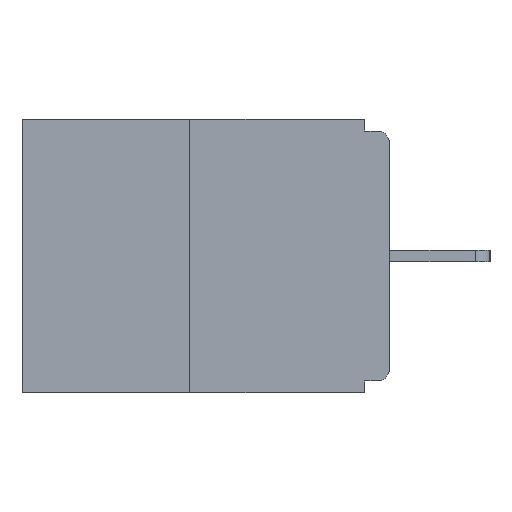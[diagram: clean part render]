
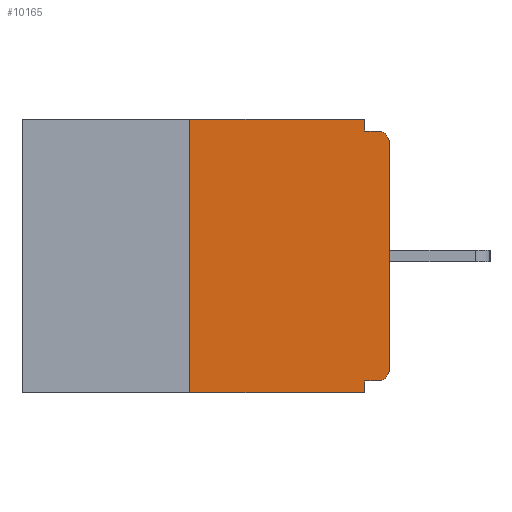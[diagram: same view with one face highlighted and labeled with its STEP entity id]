
A CAD part, left-side view. The second image highlights one B-rep face of the part: STEP entity #10165.
In plain terms, the highlighted planar face has unit normal (-1, 0, 0).
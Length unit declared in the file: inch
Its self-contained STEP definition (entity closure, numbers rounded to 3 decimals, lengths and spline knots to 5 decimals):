
#77 = CARTESIAN_POINT ( 'NONE',  ( 0., 0.031, -0.343 ) ) ;
#112 = LINE ( 'NONE', #6906, #4555 ) ;
#168 = CARTESIAN_POINT ( 'NONE',  ( 0., 0.015, -0.03 ) ) ;
#309 = EDGE_CURVE ( 'NONE', #3891, #2031, #1038, .T. ) ;
#332 = DIRECTION ( 'NONE',  ( 0., 0., -1. ) ) ;
#1038 = LINE ( 'NONE', #4502, #12500 ) ;
#1182 = DIRECTION ( 'NONE',  ( 0., 0., -1. ) ) ;
#1231 = LINE ( 'NONE', #9130, #6638 ) ;
#1246 = EDGE_CURVE ( 'NONE', #8167, #6120, #4757, .T. ) ;
#1409 = ORIENTED_EDGE ( 'NONE', *, *, #309, .F. ) ;
#1579 = CARTESIAN_POINT ( 'NONE',  ( 0., 0., -0.328 ) ) ;
#1646 = VECTOR ( 'NONE', #14149, 39.37008 ) ;
#2031 = VERTEX_POINT ( 'NONE', #12581 ) ;
#2086 = CARTESIAN_POINT ( 'NONE',  ( 0., 0., -0.015 ) ) ;
#2393 = CARTESIAN_POINT ( 'NONE',  ( 0., 0.25, 0. ) ) ;
#2435 = ORIENTED_EDGE ( 'NONE', *, *, #1246, .T. ) ;
#2538 = DIRECTION ( 'NONE',  ( 0., 0., -1. ) ) ;
#2892 = EDGE_CURVE ( 'NONE', #6120, #8867, #10414, .T. ) ;
#3106 = LINE ( 'NONE', #6288, #1646 ) ;
#3425 = CARTESIAN_POINT ( 'NONE',  ( 0., 0.015, -0.328 ) ) ;
#3812 = EDGE_CURVE ( 'NONE', #9944, #8167, #5420, .T. ) ;
#3814 = ORIENTED_EDGE ( 'NONE', *, *, #2892, .T. ) ;
#3891 = VERTEX_POINT ( 'NONE', #12996 ) ;
#4291 = CARTESIAN_POINT ( 'NONE',  ( 0., 0.25, -0.343 ) ) ;
#4444 = CARTESIAN_POINT ( 'NONE',  ( 0., 0.46, 0. ) ) ;
#4502 = CARTESIAN_POINT ( 'NONE',  ( 0., 0.031, 0. ) ) ;
#4518 = ORIENTED_EDGE ( 'NONE', *, *, #3812, .T. ) ;
#4555 = VECTOR ( 'NONE', #4827, 39.37008 ) ;
#4739 = AXIS2_PLACEMENT_3D ( 'NONE', #168, #8147, #2538 ) ;
#4757 = LINE ( 'NONE', #8087, #12994 ) ;
#4827 = DIRECTION ( 'NONE',  ( 0., -1., 0. ) ) ;
#4846 = CARTESIAN_POINT ( 'NONE',  ( 0., 0.031, -0.328 ) ) ;
#5420 = CIRCLE ( 'NONE', #14435, 0.015 ) ;
#5537 = EDGE_CURVE ( 'NONE', #14638, #13087, #3106, .T. ) ;
#6006 = VECTOR ( 'NONE', #13215, 39.37008 ) ;
#6070 = ORIENTED_EDGE ( 'NONE', *, *, #12764, .T. ) ;
#6120 = VERTEX_POINT ( 'NONE', #12477 ) ;
#6288 = CARTESIAN_POINT ( 'NONE',  ( 0., 0.25, 0. ) ) ;
#6302 = DIRECTION ( 'NONE',  ( -1., 0., 0. ) ) ;
#6491 = ORIENTED_EDGE ( 'NONE', *, *, #8341, .F. ) ;
#6595 = LINE ( 'NONE', #4444, #7169 ) ;
#6638 = VECTOR ( 'NONE', #332, 39.37008 ) ;
#6906 = CARTESIAN_POINT ( 'NONE',  ( 0., 0.46, -0.343 ) ) ;
#7099 = LINE ( 'NONE', #1579, #7656 ) ;
#7163 = EDGE_LOOP ( 'NONE', ( #13768, #14535, #6070, #6491, #8453, #4518, #2435, #3814, #11019, #1409 ) ) ;
#7169 = VECTOR ( 'NONE', #13229, 39.37008 ) ;
#7449 = VERTEX_POINT ( 'NONE', #77 ) ;
#7656 = VECTOR ( 'NONE', #13795, 39.37008 ) ;
#8087 = CARTESIAN_POINT ( 'NONE',  ( 0., 0., 0. ) ) ;
#8147 = DIRECTION ( 'NONE',  ( -1., 0., 0. ) ) ;
#8167 = VERTEX_POINT ( 'NONE', #11284 ) ;
#8341 = EDGE_CURVE ( 'NONE', #12434, #7449, #1231, .T. ) ;
#8368 = CARTESIAN_POINT ( 'NONE',  ( 0., 0.015, -0.015 ) ) ;
#8437 = DIRECTION ( 'NONE',  ( 1., 0., 0. ) ) ;
#8453 = ORIENTED_EDGE ( 'NONE', *, *, #14336, .F. ) ;
#8660 = DIRECTION ( 'NONE',  ( 0., 0., -1. ) ) ;
#8867 = VERTEX_POINT ( 'NONE', #8368 ) ;
#9130 = CARTESIAN_POINT ( 'NONE',  ( 0., 0.031, -0.343 ) ) ;
#9266 = DIRECTION ( 'NONE',  ( 0., 0., 1. ) ) ;
#9791 = PLANE ( 'NONE',  #14274 ) ;
#9862 = CARTESIAN_POINT ( 'NONE',  ( 0., 0.015, -0.313 ) ) ;
#9944 = VERTEX_POINT ( 'NONE', #3425 ) ;
#10165 = ADVANCED_FACE ( 'NONE', ( #14331 ), #9791, .F. ) ;
#10414 = CIRCLE ( 'NONE', #4739, 0.015 ) ;
#10960 = LINE ( 'NONE', #2086, #6006 ) ;
#11019 = ORIENTED_EDGE ( 'NONE', *, *, #13344, .F. ) ;
#11284 = CARTESIAN_POINT ( 'NONE',  ( 0., 0., -0.313 ) ) ;
#11728 = DIRECTION ( 'NONE',  ( 0., 0., -1. ) ) ;
#11867 = EDGE_CURVE ( 'NONE', #13087, #3891, #6595, .T. ) ;
#12434 = VERTEX_POINT ( 'NONE', #4846 ) ;
#12477 = CARTESIAN_POINT ( 'NONE',  ( 0., 0., -0.03 ) ) ;
#12500 = VECTOR ( 'NONE', #1182, 39.37008 ) ;
#12581 = CARTESIAN_POINT ( 'NONE',  ( 0., 0.031, -0.015 ) ) ;
#12764 = EDGE_CURVE ( 'NONE', #14638, #7449, #112, .T. ) ;
#12994 = VECTOR ( 'NONE', #9266, 39.37008 ) ;
#12996 = CARTESIAN_POINT ( 'NONE',  ( 0., 0.031, 0. ) ) ;
#13087 = VERTEX_POINT ( 'NONE', #2393 ) ;
#13215 = DIRECTION ( 'NONE',  ( 0., -1., 0. ) ) ;
#13229 = DIRECTION ( 'NONE',  ( 0., -1., 0. ) ) ;
#13344 = EDGE_CURVE ( 'NONE', #2031, #8867, #10960, .T. ) ;
#13768 = ORIENTED_EDGE ( 'NONE', *, *, #11867, .F. ) ;
#13795 = DIRECTION ( 'NONE',  ( 0., 1., 0. ) ) ;
#14095 = CARTESIAN_POINT ( 'NONE',  ( 0., 0.46, 0. ) ) ;
#14149 = DIRECTION ( 'NONE',  ( 0., 0., 1. ) ) ;
#14274 = AXIS2_PLACEMENT_3D ( 'NONE', #14095, #8437, #11728 ) ;
#14331 = FACE_OUTER_BOUND ( 'NONE', #7163, .T. ) ;
#14336 = EDGE_CURVE ( 'NONE', #9944, #12434, #7099, .T. ) ;
#14435 = AXIS2_PLACEMENT_3D ( 'NONE', #9862, #6302, #8660 ) ;
#14535 = ORIENTED_EDGE ( 'NONE', *, *, #5537, .F. ) ;
#14638 = VERTEX_POINT ( 'NONE', #4291 ) ;
